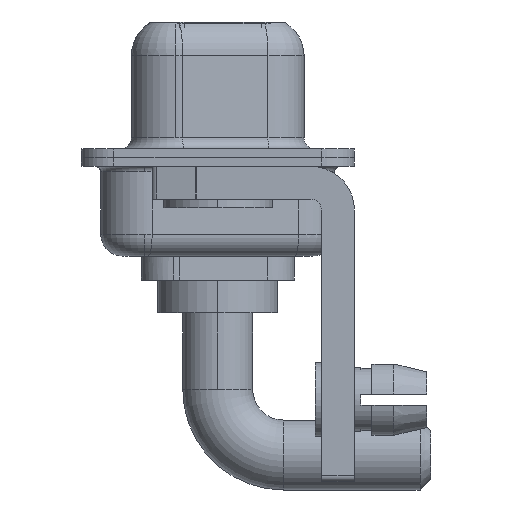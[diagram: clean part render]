
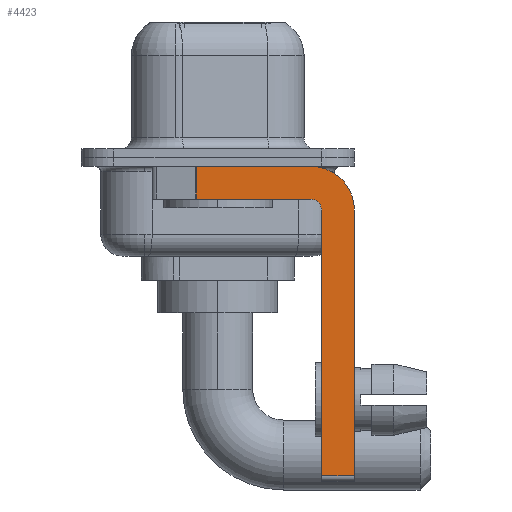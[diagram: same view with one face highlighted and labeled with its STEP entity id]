
A CAD part, left-side view. The second image highlights one B-rep face of the part: STEP entity #4423.
In plain terms, the highlighted planar face has unit normal (-1, 0, 0).
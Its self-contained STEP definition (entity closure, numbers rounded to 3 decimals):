
#124 = EDGE_CURVE ( 'NONE', #10246, #7088, #13105, .T. ) ;
#493 = VECTOR ( 'NONE', #5748, 1000. ) ;
#672 = EDGE_CURVE ( 'NONE', #4161, #9744, #15238, .T. ) ;
#987 = ORIENTED_EDGE ( 'NONE', *, *, #672, .F. ) ;
#1101 = FACE_OUTER_BOUND ( 'NONE', #4781, .T. ) ;
#1965 = EDGE_CURVE ( 'NONE', #11751, #3072, #13751, .T. ) ;
#2335 = CARTESIAN_POINT ( 'NONE',  ( -2.9, -4.75, -2.4 ) ) ;
#2717 = DIRECTION ( 'NONE',  ( 0., 0., 1. ) ) ;
#2866 = CARTESIAN_POINT ( 'NONE',  ( -2.9, -4.25, -14.55 ) ) ;
#2962 = ORIENTED_EDGE ( 'NONE', *, *, #1965, .T. ) ;
#3072 = VERTEX_POINT ( 'NONE', #8695 ) ;
#3163 = CARTESIAN_POINT ( 'NONE',  ( -2.9, -4.25, -1.9 ) ) ;
#3230 = DIRECTION ( 'NONE',  ( 0., 1., 0. ) ) ;
#3406 = VERTEX_POINT ( 'NONE', #2335 ) ;
#3554 = DIRECTION ( 'NONE',  ( 1., 0., 0. ) ) ;
#3923 = CARTESIAN_POINT ( 'NONE',  ( -2.9, 0.978, -0.4 ) ) ;
#4161 = VERTEX_POINT ( 'NONE', #9277 ) ;
#4214 = DIRECTION ( 'NONE',  ( 0., 0., 1. ) ) ;
#4336 = ORIENTED_EDGE ( 'NONE', *, *, #124, .T. ) ;
#4423 = ADVANCED_FACE ( 'NONE', ( #1101 ), #14425, .F. ) ;
#4579 = CARTESIAN_POINT ( 'NONE',  ( -2.9, -4.25, -1.9 ) ) ;
#4781 = EDGE_LOOP ( 'NONE', ( #10019, #4336, #11437, #6972, #11410, #2962, #11699, #987 ) ) ;
#5387 = EDGE_CURVE ( 'NONE', #11751, #3406, #14777, .T. ) ;
#5748 = DIRECTION ( 'NONE',  ( 0., 0., -1. ) ) ;
#6045 = CARTESIAN_POINT ( 'NONE',  ( -2.9, 3., -0.4 ) ) ;
#6476 = LINE ( 'NONE', #11373, #15271 ) ;
#6760 = CARTESIAN_POINT ( 'NONE',  ( -2.9, -4.25, -2.4 ) ) ;
#6968 = VECTOR ( 'NONE', #15095, 1000. ) ;
#6972 = ORIENTED_EDGE ( 'NONE', *, *, #7206, .F. ) ;
#7077 = VECTOR ( 'NONE', #10780, 1000. ) ;
#7088 = VERTEX_POINT ( 'NONE', #13577 ) ;
#7151 = LINE ( 'NONE', #6045, #7077 ) ;
#7206 = EDGE_CURVE ( 'NONE', #3406, #13451, #14482, .T. ) ;
#7284 = VECTOR ( 'NONE', #2717, 1000. ) ;
#7444 = AXIS2_PLACEMENT_3D ( 'NONE', #8236, #3554, #8159 ) ;
#8159 = DIRECTION ( 'NONE',  ( 0., 0., -1. ) ) ;
#8236 = CARTESIAN_POINT ( 'NONE',  ( -2.9, -4.25, -2.4 ) ) ;
#8606 = CARTESIAN_POINT ( 'NONE',  ( -2.9, -4.75, -14.55 ) ) ;
#8695 = CARTESIAN_POINT ( 'NONE',  ( -2.9, -6.25, -14.55 ) ) ;
#8734 = CARTESIAN_POINT ( 'NONE',  ( -2.9, -4.75, -14.8 ) ) ;
#8890 = AXIS2_PLACEMENT_3D ( 'NONE', #9282, #13159, #13091 ) ;
#9226 = EDGE_CURVE ( 'NONE', #13451, #7088, #10738, .T. ) ;
#9277 = CARTESIAN_POINT ( 'NONE',  ( -2.9, -4.25, -0.4 ) ) ;
#9282 = CARTESIAN_POINT ( 'NONE',  ( -2.9, -4.25, -2.4 ) ) ;
#9744 = VERTEX_POINT ( 'NONE', #10267 ) ;
#10019 = ORIENTED_EDGE ( 'NONE', *, *, #15600, .F. ) ;
#10219 = DIRECTION ( 'NONE',  ( -1., 0., 0. ) ) ;
#10246 = VERTEX_POINT ( 'NONE', #3923 ) ;
#10259 = EDGE_CURVE ( 'NONE', #9744, #3072, #6476, .T. ) ;
#10267 = CARTESIAN_POINT ( 'NONE',  ( -2.9, -6.25, -2.4 ) ) ;
#10416 = AXIS2_PLACEMENT_3D ( 'NONE', #6760, #10219, #4214 ) ;
#10738 = LINE ( 'NONE', #4579, #14280 ) ;
#10780 = DIRECTION ( 'NONE',  ( 0., -1., 0. ) ) ;
#11373 = CARTESIAN_POINT ( 'NONE',  ( -2.9, -6.25, -2.4 ) ) ;
#11410 = ORIENTED_EDGE ( 'NONE', *, *, #5387, .F. ) ;
#11437 = ORIENTED_EDGE ( 'NONE', *, *, #9226, .F. ) ;
#11699 = ORIENTED_EDGE ( 'NONE', *, *, #10259, .F. ) ;
#11751 = VERTEX_POINT ( 'NONE', #8606 ) ;
#13091 = DIRECTION ( 'NONE',  ( 0., 0., -1. ) ) ;
#13105 = LINE ( 'NONE', #14228, #493 ) ;
#13159 = DIRECTION ( 'NONE',  ( 1., 0., 0. ) ) ;
#13451 = VERTEX_POINT ( 'NONE', #3163 ) ;
#13577 = CARTESIAN_POINT ( 'NONE',  ( -2.9, 0.978, -1.9 ) ) ;
#13751 = LINE ( 'NONE', #2866, #6968 ) ;
#14228 = CARTESIAN_POINT ( 'NONE',  ( -2.9, 0.978, -1.9 ) ) ;
#14280 = VECTOR ( 'NONE', #3230, 1000. ) ;
#14425 = PLANE ( 'NONE',  #7444 ) ;
#14482 = CIRCLE ( 'NONE', #10416, 0.5 ) ;
#14777 = LINE ( 'NONE', #8734, #7284 ) ;
#15032 = DIRECTION ( 'NONE',  ( 0., 0., -1. ) ) ;
#15095 = DIRECTION ( 'NONE',  ( 0., -1., 0. ) ) ;
#15238 = CIRCLE ( 'NONE', #8890, 2. ) ;
#15271 = VECTOR ( 'NONE', #15032, 1000. ) ;
#15600 = EDGE_CURVE ( 'NONE', #10246, #4161, #7151, .T. ) ;
